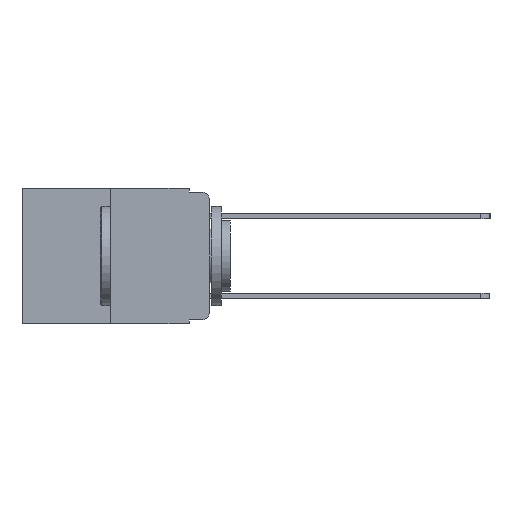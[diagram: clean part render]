
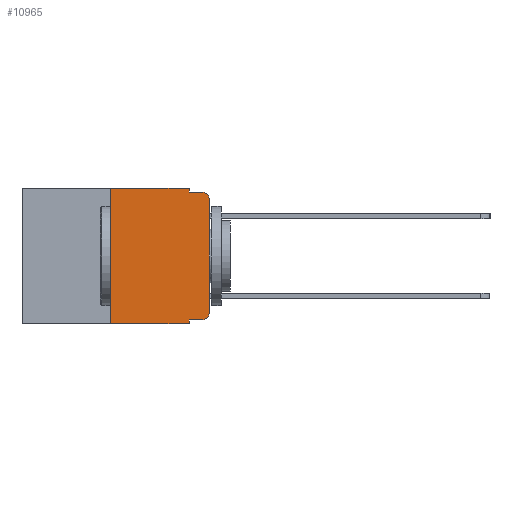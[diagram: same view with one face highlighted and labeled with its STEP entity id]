
A CAD part, left-side view. The second image highlights one B-rep face of the part: STEP entity #10965.
In plain terms, the highlighted planar face has unit normal (-1, 0, 0).
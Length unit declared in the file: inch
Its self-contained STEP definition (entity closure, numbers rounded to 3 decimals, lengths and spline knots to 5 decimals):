
#463 = DIRECTION ( 'NONE',  ( -1., 0., 0. ) ) ;
#559 = CARTESIAN_POINT ( 'NONE',  ( 0., 0.02, -0.03 ) ) ;
#815 = DIRECTION ( 'NONE',  ( 0., -1., 0. ) ) ;
#863 = LINE ( 'NONE', #7514, #6276 ) ;
#991 = VERTEX_POINT ( 'NONE', #5275 ) ;
#1178 = LINE ( 'NONE', #5688, #6547 ) ;
#1426 = VERTEX_POINT ( 'NONE', #5379 ) ;
#1552 = CARTESIAN_POINT ( 'NONE',  ( 0., 0.051, 0. ) ) ;
#1586 = VECTOR ( 'NONE', #9574, 39.37008 ) ;
#1803 = PLANE ( 'NONE',  #5766 ) ;
#1967 = CARTESIAN_POINT ( 'NONE',  ( 0., 0.051, -0.01 ) ) ;
#2157 = EDGE_CURVE ( 'NONE', #9900, #6211, #3171, .T. ) ;
#2367 = ORIENTED_EDGE ( 'NONE', *, *, #4210, .T. ) ;
#2442 = VECTOR ( 'NONE', #815, 39.37008 ) ;
#2446 = DIRECTION ( 'NONE',  ( -1., 0., 0. ) ) ;
#2793 = LINE ( 'NONE', #1967, #2442 ) ;
#2975 = DIRECTION ( 'NONE',  ( 0., 0., -1. ) ) ;
#3036 = VERTEX_POINT ( 'NONE', #11679 ) ;
#3118 = ORIENTED_EDGE ( 'NONE', *, *, #5875, .T. ) ;
#3171 = CIRCLE ( 'NONE', #10044, 0.02 ) ;
#3185 = EDGE_CURVE ( 'NONE', #8715, #991, #4021, .T. ) ;
#3315 = CARTESIAN_POINT ( 'NONE',  ( 0., 0.02, -0.333 ) ) ;
#3471 = ORIENTED_EDGE ( 'NONE', *, *, #3185, .F. ) ;
#3633 = EDGE_CURVE ( 'NONE', #991, #6211, #2793, .T. ) ;
#3782 = AXIS2_PLACEMENT_3D ( 'NONE', #8808, #2446, #9731 ) ;
#3939 = VERTEX_POINT ( 'NONE', #9661 ) ;
#4003 = ORIENTED_EDGE ( 'NONE', *, *, #3633, .F. ) ;
#4021 = LINE ( 'NONE', #1552, #6264 ) ;
#4210 = EDGE_CURVE ( 'NONE', #3036, #9900, #863, .T. ) ;
#4309 = DIRECTION ( 'NONE',  ( 0., 0., 1. ) ) ;
#4617 = DIRECTION ( 'NONE',  ( 0., 0., -1. ) ) ;
#4692 = LINE ( 'NONE', #10560, #1586 ) ;
#5063 = CARTESIAN_POINT ( 'NONE',  ( 0., 0.473, 0. ) ) ;
#5172 = VECTOR ( 'NONE', #11059, 39.37008 ) ;
#5275 = CARTESIAN_POINT ( 'NONE',  ( 0., 0.051, -0.01 ) ) ;
#5379 = CARTESIAN_POINT ( 'NONE',  ( 0., 0.25, 0. ) ) ;
#5421 = FACE_OUTER_BOUND ( 'NONE', #6030, .T. ) ;
#5441 = DIRECTION ( 'NONE',  ( 0., 0., -1. ) ) ;
#5546 = VERTEX_POINT ( 'NONE', #10888 ) ;
#5577 = ORIENTED_EDGE ( 'NONE', *, *, #6888, .F. ) ;
#5681 = LINE ( 'NONE', #13394, #10293 ) ;
#5688 = CARTESIAN_POINT ( 'NONE',  ( 0., 0.051, -0.333 ) ) ;
#5766 = AXIS2_PLACEMENT_3D ( 'NONE', #13013, #9250, #2975 ) ;
#5815 = EDGE_CURVE ( 'NONE', #5546, #9550, #4692, .T. ) ;
#5843 = LINE ( 'NONE', #5063, #12934 ) ;
#5875 = EDGE_CURVE ( 'NONE', #12383, #3036, #9411, .T. ) ;
#6001 = CARTESIAN_POINT ( 'NONE',  ( 0., 0., -0.03 ) ) ;
#6030 = EDGE_LOOP ( 'NONE', ( #2367, #7678, #4003, #3471, #12428, #5577, #11992, #9729, #8138, #3118 ) ) ;
#6211 = VERTEX_POINT ( 'NONE', #11439 ) ;
#6263 = EDGE_CURVE ( 'NONE', #3939, #12383, #1178, .T. ) ;
#6264 = VECTOR ( 'NONE', #5441, 39.37008 ) ;
#6276 = VECTOR ( 'NONE', #4309, 39.37008 ) ;
#6547 = VECTOR ( 'NONE', #9635, 39.37008 ) ;
#6703 = CARTESIAN_POINT ( 'NONE',  ( 0., 0.051, -0.343 ) ) ;
#6740 = EDGE_CURVE ( 'NONE', #3939, #9550, #5681, .T. ) ;
#6888 = EDGE_CURVE ( 'NONE', #5546, #1426, #12946, .T. ) ;
#7131 = CARTESIAN_POINT ( 'NONE',  ( 0., 0.051, 0. ) ) ;
#7169 = EDGE_CURVE ( 'NONE', #1426, #8715, #5843, .T. ) ;
#7514 = CARTESIAN_POINT ( 'NONE',  ( 0., 0., 0. ) ) ;
#7678 = ORIENTED_EDGE ( 'NONE', *, *, #2157, .T. ) ;
#8138 = ORIENTED_EDGE ( 'NONE', *, *, #6263, .T. ) ;
#8715 = VERTEX_POINT ( 'NONE', #7131 ) ;
#8808 = CARTESIAN_POINT ( 'NONE',  ( 0., 0.02, -0.313 ) ) ;
#9250 = DIRECTION ( 'NONE',  ( 1., 0., 0. ) ) ;
#9411 = CIRCLE ( 'NONE', #3782, 0.02 ) ;
#9550 = VERTEX_POINT ( 'NONE', #6703 ) ;
#9574 = DIRECTION ( 'NONE',  ( 0., -1., 0. ) ) ;
#9635 = DIRECTION ( 'NONE',  ( 0., -1., 0. ) ) ;
#9661 = CARTESIAN_POINT ( 'NONE',  ( 0., 0.051, -0.333 ) ) ;
#9729 = ORIENTED_EDGE ( 'NONE', *, *, #6740, .F. ) ;
#9731 = DIRECTION ( 'NONE',  ( 0., 0., -1. ) ) ;
#9900 = VERTEX_POINT ( 'NONE', #6001 ) ;
#10044 = AXIS2_PLACEMENT_3D ( 'NONE', #559, #463, #11485 ) ;
#10103 = CARTESIAN_POINT ( 'NONE',  ( 0., 0.25, 0. ) ) ;
#10293 = VECTOR ( 'NONE', #4617, 39.37008 ) ;
#10560 = CARTESIAN_POINT ( 'NONE',  ( 0., 0.473, -0.343 ) ) ;
#10888 = CARTESIAN_POINT ( 'NONE',  ( 0., 0.25, -0.343 ) ) ;
#10965 = ADVANCED_FACE ( 'NONE', ( #5421 ), #1803, .F. ) ;
#11059 = DIRECTION ( 'NONE',  ( 0., 0., 1. ) ) ;
#11439 = CARTESIAN_POINT ( 'NONE',  ( 0., 0.02, -0.01 ) ) ;
#11485 = DIRECTION ( 'NONE',  ( 0., 0., -1. ) ) ;
#11679 = CARTESIAN_POINT ( 'NONE',  ( 0., 0., -0.313 ) ) ;
#11992 = ORIENTED_EDGE ( 'NONE', *, *, #5815, .T. ) ;
#12383 = VERTEX_POINT ( 'NONE', #3315 ) ;
#12428 = ORIENTED_EDGE ( 'NONE', *, *, #7169, .F. ) ;
#12876 = DIRECTION ( 'NONE',  ( 0., -1., 0. ) ) ;
#12934 = VECTOR ( 'NONE', #12876, 39.37008 ) ;
#12946 = LINE ( 'NONE', #10103, #5172 ) ;
#13013 = CARTESIAN_POINT ( 'NONE',  ( 0., 0.473, 0. ) ) ;
#13394 = CARTESIAN_POINT ( 'NONE',  ( 0., 0.051, 0. ) ) ;
